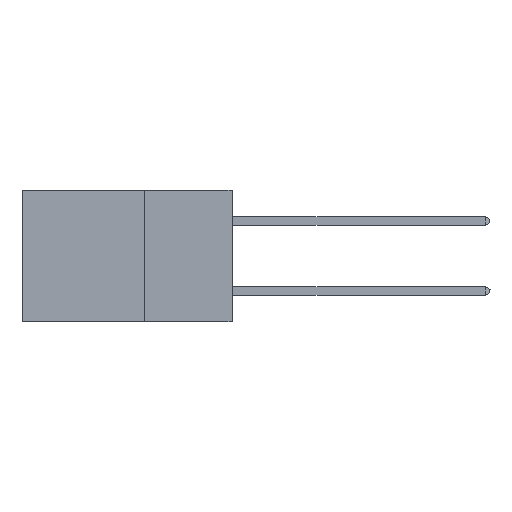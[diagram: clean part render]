
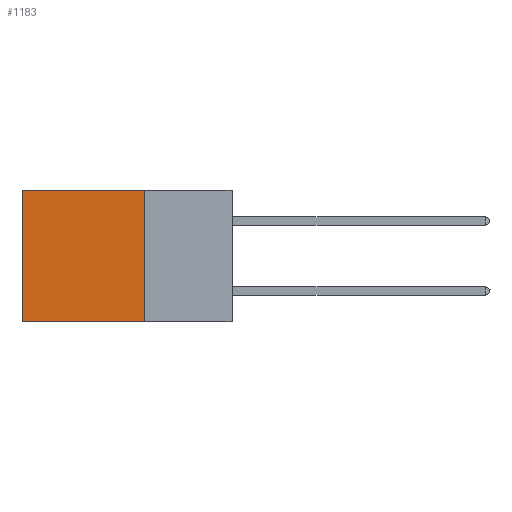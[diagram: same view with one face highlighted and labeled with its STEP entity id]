
A CAD part, left-side view. The second image highlights one B-rep face of the part: STEP entity #1183.
In plain terms, the highlighted planar face has unit normal (-1, 0, 0).
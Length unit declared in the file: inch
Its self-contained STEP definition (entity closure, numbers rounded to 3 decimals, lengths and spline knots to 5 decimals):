
#365 = FACE_OUTER_BOUND ( 'NONE', #6789, .T. ) ;
#570 = AXIS2_PLACEMENT_3D ( 'NONE', #18354, #900, #11079 ) ;
#900 = DIRECTION ( 'NONE',  ( 1., 0., 0. ) ) ;
#1183 = ADVANCED_FACE ( 'NONE', ( #365 ), #8132, .F. ) ;
#1481 = EDGE_CURVE ( 'NONE', #13117, #17893, #13950, .T. ) ;
#1870 = DIRECTION ( 'NONE',  ( 0., 0., -1. ) ) ;
#3155 = CARTESIAN_POINT ( 'NONE',  ( 0.2875, 0.25, -0.375 ) ) ;
#3335 = CARTESIAN_POINT ( 'NONE',  ( 0.2875, 0.25, -0.375 ) ) ;
#3718 = EDGE_CURVE ( 'NONE', #13862, #15419, #8464, .T. ) ;
#4238 = ORIENTED_EDGE ( 'NONE', *, *, #3718, .F. ) ;
#4565 = DIRECTION ( 'NONE',  ( 0., 1., 0. ) ) ;
#6695 = LINE ( 'NONE', #3155, #14662 ) ;
#6789 = EDGE_LOOP ( 'NONE', ( #11559, #7897, #4238, #10376 ) ) ;
#7442 = CARTESIAN_POINT ( 'NONE',  ( 0.2875, 0.6, -0.375 ) ) ;
#7897 = ORIENTED_EDGE ( 'NONE', *, *, #14935, .F. ) ;
#8132 = PLANE ( 'NONE',  #570 ) ;
#8256 = EDGE_CURVE ( 'NONE', #13862, #13117, #17469, .T. ) ;
#8464 = LINE ( 'NONE', #18590, #11877 ) ;
#10109 = VECTOR ( 'NONE', #1870, 39.37008 ) ;
#10376 = ORIENTED_EDGE ( 'NONE', *, *, #8256, .T. ) ;
#11079 = DIRECTION ( 'NONE',  ( 0., 0., -1. ) ) ;
#11559 = ORIENTED_EDGE ( 'NONE', *, *, #1481, .T. ) ;
#11877 = VECTOR ( 'NONE', #15641, 39.37008 ) ;
#12209 = VECTOR ( 'NONE', #4565, 39.37008 ) ;
#13117 = VERTEX_POINT ( 'NONE', #17223 ) ;
#13136 = CARTESIAN_POINT ( 'NONE',  ( 0.2875, 0.25, 0. ) ) ;
#13304 = DIRECTION ( 'NONE',  ( 0., 1., 0. ) ) ;
#13862 = VERTEX_POINT ( 'NONE', #15881 ) ;
#13950 = LINE ( 'NONE', #14867, #10109 ) ;
#14662 = VECTOR ( 'NONE', #13304, 39.37008 ) ;
#14867 = CARTESIAN_POINT ( 'NONE',  ( 0.2875, 0.6, -0.375 ) ) ;
#14935 = EDGE_CURVE ( 'NONE', #15419, #17893, #6695, .T. ) ;
#15419 = VERTEX_POINT ( 'NONE', #3335 ) ;
#15641 = DIRECTION ( 'NONE',  ( 0., 0., -1. ) ) ;
#15881 = CARTESIAN_POINT ( 'NONE',  ( 0.2875, 0.25, 0. ) ) ;
#17223 = CARTESIAN_POINT ( 'NONE',  ( 0.2875, 0.6, 0. ) ) ;
#17469 = LINE ( 'NONE', #13136, #12209 ) ;
#17893 = VERTEX_POINT ( 'NONE', #7442 ) ;
#18354 = CARTESIAN_POINT ( 'NONE',  ( 0.2875, 0.25, -0.375 ) ) ;
#18590 = CARTESIAN_POINT ( 'NONE',  ( 0.2875, 0.25, -0.375 ) ) ;
